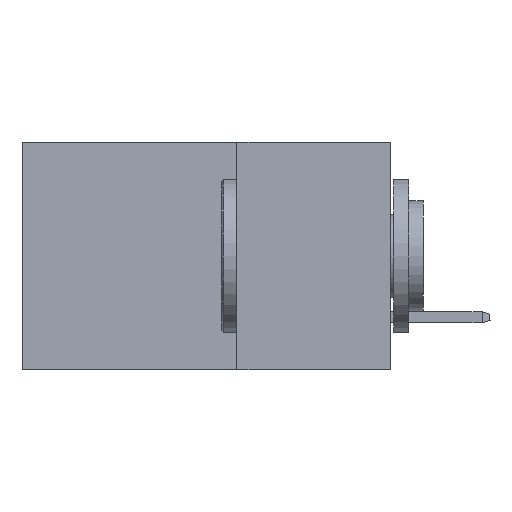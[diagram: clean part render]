
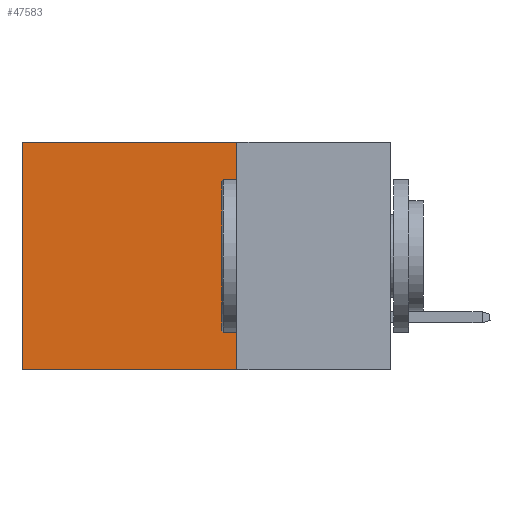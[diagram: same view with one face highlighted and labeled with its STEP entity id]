
A CAD part, left-side view. The second image highlights one B-rep face of the part: STEP entity #47583.
In plain terms, the highlighted planar face has unit normal (-1, 0, 0).
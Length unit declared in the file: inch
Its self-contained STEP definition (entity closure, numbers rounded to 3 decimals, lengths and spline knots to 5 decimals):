
#242 = EDGE_CURVE ( 'NONE', #20862, #38190, #2635, .T. ) ;
#2635 = LINE ( 'NONE', #36458, #25507 ) ;
#2741 = VECTOR ( 'NONE', #39103, 39.37008 ) ;
#3365 = LINE ( 'NONE', #46669, #2741 ) ;
#3547 = EDGE_CURVE ( 'NONE', #37409, #38190, #41421, .T. ) ;
#3753 = DIRECTION ( 'NONE',  ( 0., 0., -1. ) ) ;
#3890 = DIRECTION ( 'NONE',  ( 1., 0., 0. ) ) ;
#5968 = ORIENTED_EDGE ( 'NONE', *, *, #6356, .T. ) ;
#6356 = EDGE_CURVE ( 'NONE', #21758, #20862, #3365, .T. ) ;
#7274 = CARTESIAN_POINT ( 'NONE',  ( 0.2875, 0.25, -0.37 ) ) ;
#8156 = VECTOR ( 'NONE', #3753, 39.37008 ) ;
#11293 = DIRECTION ( 'NONE',  ( 0., 0., -1. ) ) ;
#19292 = CARTESIAN_POINT ( 'NONE',  ( 0.2875, 0.6, 0. ) ) ;
#20046 = CARTESIAN_POINT ( 'NONE',  ( 0.2875, 0.25, -0.37 ) ) ;
#20862 = VERTEX_POINT ( 'NONE', #19292 ) ;
#21758 = VERTEX_POINT ( 'NONE', #33153 ) ;
#23127 = CARTESIAN_POINT ( 'NONE',  ( 0.2875, 0.6, -0.37 ) ) ;
#25507 = VECTOR ( 'NONE', #28847, 39.37008 ) ;
#27604 = EDGE_CURVE ( 'NONE', #21758, #37409, #38153, .T. ) ;
#27788 = ORIENTED_EDGE ( 'NONE', *, *, #27604, .F. ) ;
#28847 = DIRECTION ( 'NONE',  ( 0., 0., -1. ) ) ;
#30936 = PLANE ( 'NONE',  #48978 ) ;
#31164 = DIRECTION ( 'NONE',  ( 0., 1., 0. ) ) ;
#32143 = ORIENTED_EDGE ( 'NONE', *, *, #242, .T. ) ;
#33028 = VECTOR ( 'NONE', #31164, 39.37008 ) ;
#33153 = CARTESIAN_POINT ( 'NONE',  ( 0.2875, 0.25, 0. ) ) ;
#34804 = CARTESIAN_POINT ( 'NONE',  ( 0.2875, 0.25, 0. ) ) ;
#36458 = CARTESIAN_POINT ( 'NONE',  ( 0.2875, 0.6, 0. ) ) ;
#37409 = VERTEX_POINT ( 'NONE', #7274 ) ;
#38153 = LINE ( 'NONE', #34804, #8156 ) ;
#38190 = VERTEX_POINT ( 'NONE', #23127 ) ;
#39103 = DIRECTION ( 'NONE',  ( 0., 1., 0. ) ) ;
#41421 = LINE ( 'NONE', #20046, #33028 ) ;
#42224 = EDGE_LOOP ( 'NONE', ( #32143, #42397, #27788, #5968 ) ) ;
#42397 = ORIENTED_EDGE ( 'NONE', *, *, #3547, .F. ) ;
#42436 = CARTESIAN_POINT ( 'NONE',  ( 0.2875, 0.25, 0. ) ) ;
#44958 = FACE_OUTER_BOUND ( 'NONE', #42224, .T. ) ;
#46669 = CARTESIAN_POINT ( 'NONE',  ( 0.2875, 0.25, 0. ) ) ;
#47583 = ADVANCED_FACE ( 'NONE', ( #44958 ), #30936, .F. ) ;
#48978 = AXIS2_PLACEMENT_3D ( 'NONE', #42436, #3890, #11293 ) ;
